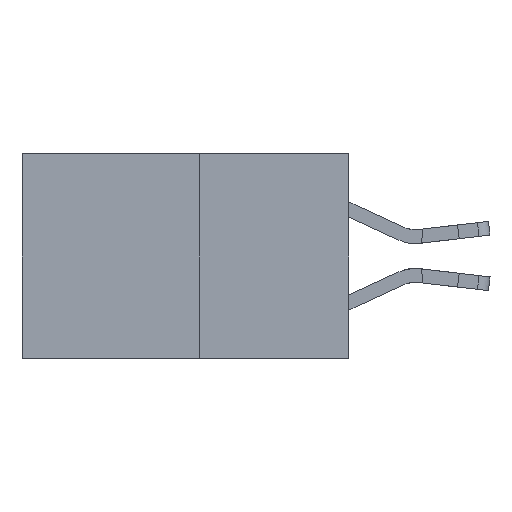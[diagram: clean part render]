
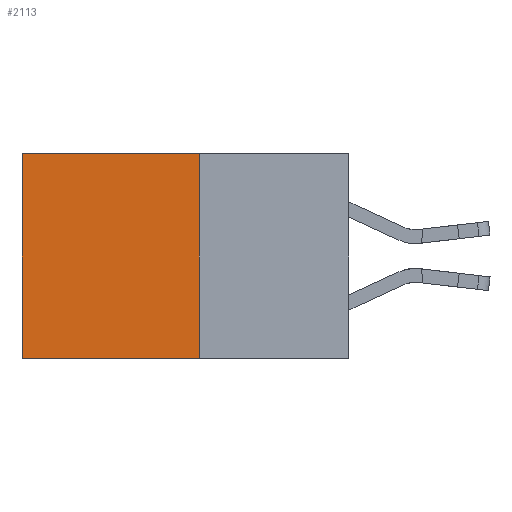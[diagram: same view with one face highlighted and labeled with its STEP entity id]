
A CAD part, left-side view. The second image highlights one B-rep face of the part: STEP entity #2113.
In plain terms, the highlighted planar face has unit normal (-1, 0, 0).
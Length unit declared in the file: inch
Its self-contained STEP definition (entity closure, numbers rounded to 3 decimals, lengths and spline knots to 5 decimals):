
#171 = DIRECTION ( 'NONE',  ( 0., 0., -1. ) ) ;
#278 = CARTESIAN_POINT ( 'NONE',  ( 0.277, 0.27, -0.37 ) ) ;
#1137 = VERTEX_POINT ( 'NONE', #15152 ) ;
#1810 = LINE ( 'NONE', #23354, #25157 ) ;
#2113 = ADVANCED_FACE ( 'NONE', ( #2766 ), #29279, .F. ) ;
#2766 = FACE_OUTER_BOUND ( 'NONE', #14618, .T. ) ;
#3216 = LINE ( 'NONE', #28367, #14597 ) ;
#3557 = VECTOR ( 'NONE', #171, 39.37008 ) ;
#4785 = VERTEX_POINT ( 'NONE', #20221 ) ;
#6855 = VERTEX_POINT ( 'NONE', #19369 ) ;
#7083 = VERTEX_POINT ( 'NONE', #21498 ) ;
#8756 = EDGE_CURVE ( 'NONE', #4785, #1137, #9579, .T. ) ;
#9579 = LINE ( 'NONE', #278, #3557 ) ;
#9783 = ORIENTED_EDGE ( 'NONE', *, *, #13312, .T. ) ;
#10183 = VECTOR ( 'NONE', #11268, 39.37008 ) ;
#10436 = DIRECTION ( 'NONE',  ( 0., 0., -1. ) ) ;
#11268 = DIRECTION ( 'NONE',  ( 0., 1., 0. ) ) ;
#12947 = ORIENTED_EDGE ( 'NONE', *, *, #8756, .F. ) ;
#13312 = EDGE_CURVE ( 'NONE', #4785, #7083, #1810, .T. ) ;
#14194 = EDGE_CURVE ( 'NONE', #7083, #6855, #3216, .T. ) ;
#14597 = VECTOR ( 'NONE', #10436, 39.37008 ) ;
#14618 = EDGE_LOOP ( 'NONE', ( #22506, #28787, #12947, #9783 ) ) ;
#15152 = CARTESIAN_POINT ( 'NONE',  ( 0.277, 0.27, -0.37 ) ) ;
#16251 = LINE ( 'NONE', #18074, #10183 ) ;
#18074 = CARTESIAN_POINT ( 'NONE',  ( 0.277, 0.27, -0.37 ) ) ;
#19369 = CARTESIAN_POINT ( 'NONE',  ( 0.277, 0.59, -0.37 ) ) ;
#20221 = CARTESIAN_POINT ( 'NONE',  ( 0.277, 0.27, 0. ) ) ;
#21498 = CARTESIAN_POINT ( 'NONE',  ( 0.277, 0.59, 0. ) ) ;
#22506 = ORIENTED_EDGE ( 'NONE', *, *, #14194, .T. ) ;
#23354 = CARTESIAN_POINT ( 'NONE',  ( 0.277, 0.27, 0. ) ) ;
#24502 = AXIS2_PLACEMENT_3D ( 'NONE', #24541, #27541, #27537 ) ;
#24541 = CARTESIAN_POINT ( 'NONE',  ( 0.277, 0.27, -0.37 ) ) ;
#25157 = VECTOR ( 'NONE', #25546, 39.37008 ) ;
#25546 = DIRECTION ( 'NONE',  ( 0., 1., 0. ) ) ;
#27537 = DIRECTION ( 'NONE',  ( 0., 0., -1. ) ) ;
#27541 = DIRECTION ( 'NONE',  ( 1., 0., 0. ) ) ;
#27979 = EDGE_CURVE ( 'NONE', #1137, #6855, #16251, .T. ) ;
#28367 = CARTESIAN_POINT ( 'NONE',  ( 0.277, 0.59, -0.37 ) ) ;
#28787 = ORIENTED_EDGE ( 'NONE', *, *, #27979, .F. ) ;
#29279 = PLANE ( 'NONE',  #24502 ) ;
